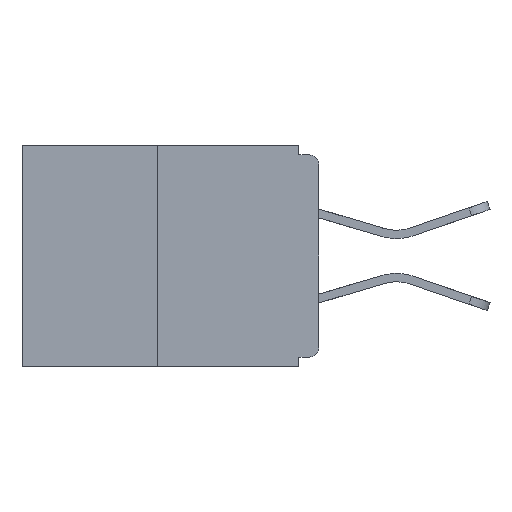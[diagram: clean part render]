
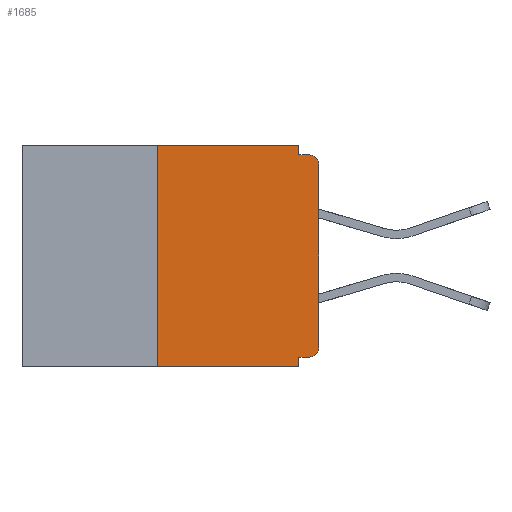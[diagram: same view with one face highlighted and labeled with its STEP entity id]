
A CAD part, left-side view. The second image highlights one B-rep face of the part: STEP entity #1685.
In plain terms, the highlighted planar face has unit normal (-1, 0, 0).
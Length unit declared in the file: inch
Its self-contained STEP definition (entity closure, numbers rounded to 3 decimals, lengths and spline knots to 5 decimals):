
#1 = DIRECTION ( 'NONE',  ( 1., 0., 0. ) ) ;
#498 = CARTESIAN_POINT ( 'NONE',  ( 0., 0.031, -0.328 ) ) ;
#543 = LINE ( 'NONE', #13136, #4789 ) ;
#752 = ORIENTED_EDGE ( 'NONE', *, *, #7247, .F. ) ;
#954 = ORIENTED_EDGE ( 'NONE', *, *, #7141, .T. ) ;
#1111 = ORIENTED_EDGE ( 'NONE', *, *, #2988, .F. ) ;
#1127 = LINE ( 'NONE', #13270, #6793 ) ;
#1144 = VECTOR ( 'NONE', #8623, 39.37008 ) ;
#1172 = LINE ( 'NONE', #13233, #12830 ) ;
#1203 = VERTEX_POINT ( 'NONE', #7945 ) ;
#1358 = AXIS2_PLACEMENT_3D ( 'NONE', #2787, #5432, #3078 ) ;
#1487 = CARTESIAN_POINT ( 'NONE',  ( 0., 0., -0.313 ) ) ;
#1506 = EDGE_CURVE ( 'NONE', #14583, #12075, #12283, .T. ) ;
#1685 = ADVANCED_FACE ( 'NONE', ( #7699 ), #14383, .F. ) ;
#1723 = LINE ( 'NONE', #12517, #11773 ) ;
#1798 = DIRECTION ( 'NONE',  ( 0., 1., 0. ) ) ;
#1858 = CARTESIAN_POINT ( 'NONE',  ( 0., 0.015, -0.313 ) ) ;
#1986 = DIRECTION ( 'NONE',  ( 0., -1., 0. ) ) ;
#2120 = ORIENTED_EDGE ( 'NONE', *, *, #9597, .T. ) ;
#2230 = VECTOR ( 'NONE', #7303, 39.37008 ) ;
#2697 = EDGE_CURVE ( 'NONE', #10191, #1203, #4186, .T. ) ;
#2787 = CARTESIAN_POINT ( 'NONE',  ( 0., 0.015, -0.03 ) ) ;
#2988 = EDGE_CURVE ( 'NONE', #10191, #6480, #7846, .T. ) ;
#3021 = DIRECTION ( 'NONE',  ( 0., 0., -1. ) ) ;
#3078 = DIRECTION ( 'NONE',  ( 0., 0., -1. ) ) ;
#3090 = ORIENTED_EDGE ( 'NONE', *, *, #2697, .T. ) ;
#3104 = DIRECTION ( 'NONE',  ( 0., -1., 0. ) ) ;
#3532 = VERTEX_POINT ( 'NONE', #12487 ) ;
#3682 = CARTESIAN_POINT ( 'NONE',  ( 0., 0.25, 0. ) ) ;
#3787 = VERTEX_POINT ( 'NONE', #498 ) ;
#4117 = CIRCLE ( 'NONE', #1358, 0.015 ) ;
#4180 = VERTEX_POINT ( 'NONE', #1487 ) ;
#4185 = LINE ( 'NONE', #11939, #1144 ) ;
#4186 = LINE ( 'NONE', #7508, #5045 ) ;
#4534 = ORIENTED_EDGE ( 'NONE', *, *, #8253, .F. ) ;
#4670 = EDGE_LOOP ( 'NONE', ( #4534, #1111, #3090, #752, #4943, #954, #2120, #6408, #10569, #10756 ) ) ;
#4789 = VECTOR ( 'NONE', #1798, 39.37008 ) ;
#4824 = EDGE_CURVE ( 'NONE', #13994, #3532, #4117, .T. ) ;
#4943 = ORIENTED_EDGE ( 'NONE', *, *, #5457, .F. ) ;
#5045 = VECTOR ( 'NONE', #9623, 39.37008 ) ;
#5432 = DIRECTION ( 'NONE',  ( -1., 0., 0. ) ) ;
#5457 = EDGE_CURVE ( 'NONE', #7410, #3787, #543, .T. ) ;
#6408 = ORIENTED_EDGE ( 'NONE', *, *, #4824, .T. ) ;
#6480 = VERTEX_POINT ( 'NONE', #3682 ) ;
#6793 = VECTOR ( 'NONE', #1986, 39.37008 ) ;
#7141 = EDGE_CURVE ( 'NONE', #7410, #4180, #10713, .T. ) ;
#7247 = EDGE_CURVE ( 'NONE', #3787, #1203, #1723, .T. ) ;
#7303 = DIRECTION ( 'NONE',  ( 0., 0., -1. ) ) ;
#7410 = VERTEX_POINT ( 'NONE', #12868 ) ;
#7508 = CARTESIAN_POINT ( 'NONE',  ( 0., 0.46, -0.343 ) ) ;
#7641 = CARTESIAN_POINT ( 'NONE',  ( 0., 0.46, 0. ) ) ;
#7699 = FACE_OUTER_BOUND ( 'NONE', #4670, .T. ) ;
#7846 = LINE ( 'NONE', #10103, #11696 ) ;
#7937 = CARTESIAN_POINT ( 'NONE',  ( 0., 0.031, 0. ) ) ;
#7945 = CARTESIAN_POINT ( 'NONE',  ( 0., 0.031, -0.343 ) ) ;
#8253 = EDGE_CURVE ( 'NONE', #6480, #14583, #1172, .T. ) ;
#8486 = AXIS2_PLACEMENT_3D ( 'NONE', #1858, #14369, #3021 ) ;
#8623 = DIRECTION ( 'NONE',  ( 0., 0., 1. ) ) ;
#9597 = EDGE_CURVE ( 'NONE', #4180, #13994, #4185, .T. ) ;
#9623 = DIRECTION ( 'NONE',  ( 0., -1., 0. ) ) ;
#9679 = EDGE_CURVE ( 'NONE', #12075, #3532, #1127, .T. ) ;
#10084 = CARTESIAN_POINT ( 'NONE',  ( 0., 0.25, -0.343 ) ) ;
#10103 = CARTESIAN_POINT ( 'NONE',  ( 0., 0.25, 0. ) ) ;
#10191 = VERTEX_POINT ( 'NONE', #10084 ) ;
#10569 = ORIENTED_EDGE ( 'NONE', *, *, #9679, .F. ) ;
#10635 = CARTESIAN_POINT ( 'NONE',  ( 0., 0.031, 0. ) ) ;
#10713 = CIRCLE ( 'NONE', #8486, 0.015 ) ;
#10756 = ORIENTED_EDGE ( 'NONE', *, *, #1506, .F. ) ;
#11352 = DIRECTION ( 'NONE',  ( 0., 0., 1. ) ) ;
#11696 = VECTOR ( 'NONE', #11352, 39.37008 ) ;
#11773 = VECTOR ( 'NONE', #13751, 39.37008 ) ;
#11851 = CARTESIAN_POINT ( 'NONE',  ( 0., 0., -0.03 ) ) ;
#11939 = CARTESIAN_POINT ( 'NONE',  ( 0., 0., 0. ) ) ;
#12075 = VERTEX_POINT ( 'NONE', #12926 ) ;
#12283 = LINE ( 'NONE', #10635, #2230 ) ;
#12487 = CARTESIAN_POINT ( 'NONE',  ( 0., 0.015, -0.015 ) ) ;
#12517 = CARTESIAN_POINT ( 'NONE',  ( 0., 0.031, -0.343 ) ) ;
#12830 = VECTOR ( 'NONE', #3104, 39.37008 ) ;
#12868 = CARTESIAN_POINT ( 'NONE',  ( 0., 0.015, -0.328 ) ) ;
#12926 = CARTESIAN_POINT ( 'NONE',  ( 0., 0.031, -0.015 ) ) ;
#13136 = CARTESIAN_POINT ( 'NONE',  ( 0., 0., -0.328 ) ) ;
#13233 = CARTESIAN_POINT ( 'NONE',  ( 0., 0.46, 0. ) ) ;
#13270 = CARTESIAN_POINT ( 'NONE',  ( 0., 0., -0.015 ) ) ;
#13751 = DIRECTION ( 'NONE',  ( 0., 0., -1. ) ) ;
#13991 = AXIS2_PLACEMENT_3D ( 'NONE', #7641, #1, #14607 ) ;
#13994 = VERTEX_POINT ( 'NONE', #11851 ) ;
#14369 = DIRECTION ( 'NONE',  ( -1., 0., 0. ) ) ;
#14383 = PLANE ( 'NONE',  #13991 ) ;
#14583 = VERTEX_POINT ( 'NONE', #7937 ) ;
#14607 = DIRECTION ( 'NONE',  ( 0., 0., -1. ) ) ;
